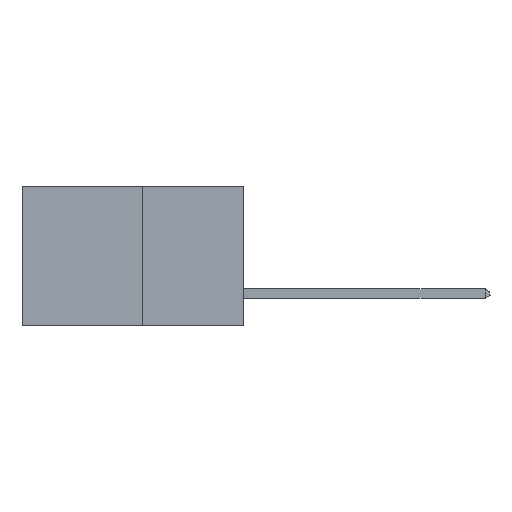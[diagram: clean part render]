
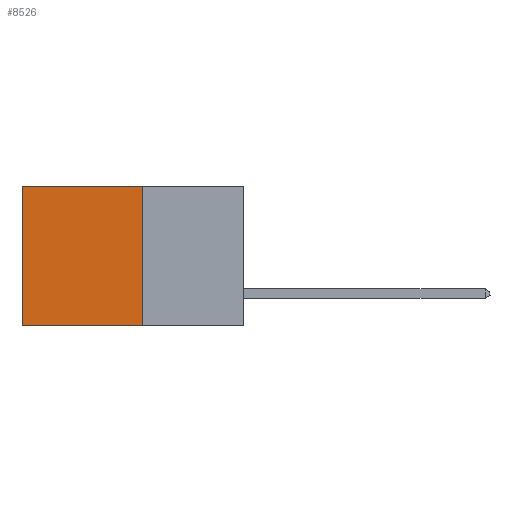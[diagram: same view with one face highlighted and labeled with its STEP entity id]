
A CAD part, left-side view. The second image highlights one B-rep face of the part: STEP entity #8526.
In plain terms, the highlighted planar face has unit normal (-1, 0, 0).
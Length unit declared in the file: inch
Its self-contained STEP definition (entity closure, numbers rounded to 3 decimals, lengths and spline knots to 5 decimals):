
#58 = FACE_OUTER_BOUND ( 'NONE', #698, .T. ) ;
#698 = EDGE_LOOP ( 'NONE', ( #18529, #2270, #14247, #18595 ) ) ;
#904 = CARTESIAN_POINT ( 'NONE',  ( 0.277, 0.27, -0.37 ) ) ;
#1356 = VECTOR ( 'NONE', #1769, 39.37008 ) ;
#1380 = VECTOR ( 'NONE', #15145, 39.37008 ) ;
#1444 = VERTEX_POINT ( 'NONE', #904 ) ;
#1769 = DIRECTION ( 'NONE',  ( 0., 0., -1. ) ) ;
#1926 = CARTESIAN_POINT ( 'NONE',  ( 0.277, 0.27, 0. ) ) ;
#1938 = CARTESIAN_POINT ( 'NONE',  ( 0.277, 0.59, -0.37 ) ) ;
#2270 = ORIENTED_EDGE ( 'NONE', *, *, #22589, .F. ) ;
#3310 = CARTESIAN_POINT ( 'NONE',  ( 0.277, 0.27, 0. ) ) ;
#6549 = AXIS2_PLACEMENT_3D ( 'NONE', #17755, #18224, #18562 ) ;
#6793 = EDGE_CURVE ( 'NONE', #23262, #1444, #14569, .T. ) ;
#8526 = ADVANCED_FACE ( 'NONE', ( #58 ), #15004, .F. ) ;
#8573 = LINE ( 'NONE', #28190, #1356 ) ;
#9759 = EDGE_CURVE ( 'NONE', #16244, #10414, #8573, .T. ) ;
#10414 = VERTEX_POINT ( 'NONE', #1938 ) ;
#14247 = ORIENTED_EDGE ( 'NONE', *, *, #6793, .F. ) ;
#14545 = CARTESIAN_POINT ( 'NONE',  ( 0.277, 0.27, -0.37 ) ) ;
#14569 = LINE ( 'NONE', #14545, #26369 ) ;
#15004 = PLANE ( 'NONE',  #6549 ) ;
#15145 = DIRECTION ( 'NONE',  ( 0., 1., 0. ) ) ;
#16244 = VERTEX_POINT ( 'NONE', #20791 ) ;
#17755 = CARTESIAN_POINT ( 'NONE',  ( 0.277, 0.27, -0.37 ) ) ;
#18224 = DIRECTION ( 'NONE',  ( 1., 0., 0. ) ) ;
#18529 = ORIENTED_EDGE ( 'NONE', *, *, #9759, .T. ) ;
#18562 = DIRECTION ( 'NONE',  ( 0., 0., -1. ) ) ;
#18595 = ORIENTED_EDGE ( 'NONE', *, *, #23018, .T. ) ;
#18955 = DIRECTION ( 'NONE',  ( 0., 0., -1. ) ) ;
#19520 = VECTOR ( 'NONE', #25356, 39.37008 ) ;
#20791 = CARTESIAN_POINT ( 'NONE',  ( 0.277, 0.59, 0. ) ) ;
#22589 = EDGE_CURVE ( 'NONE', #1444, #10414, #25514, .T. ) ;
#23018 = EDGE_CURVE ( 'NONE', #23262, #16244, #26154, .T. ) ;
#23262 = VERTEX_POINT ( 'NONE', #1926 ) ;
#23998 = CARTESIAN_POINT ( 'NONE',  ( 0.277, 0.27, -0.37 ) ) ;
#25356 = DIRECTION ( 'NONE',  ( 0., 1., 0. ) ) ;
#25514 = LINE ( 'NONE', #23998, #1380 ) ;
#26154 = LINE ( 'NONE', #3310, #19520 ) ;
#26369 = VECTOR ( 'NONE', #18955, 39.37008 ) ;
#28190 = CARTESIAN_POINT ( 'NONE',  ( 0.277, 0.59, -0.37 ) ) ;
